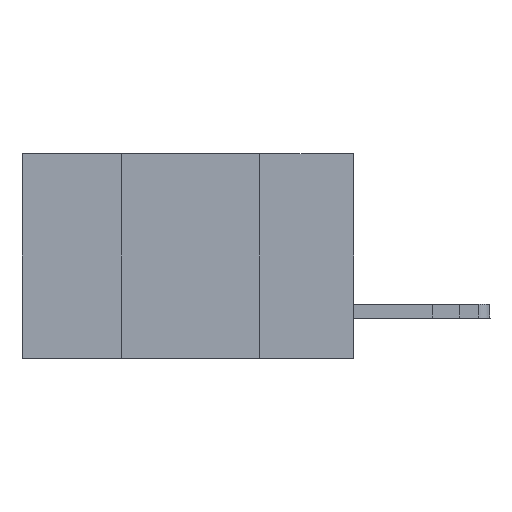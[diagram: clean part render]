
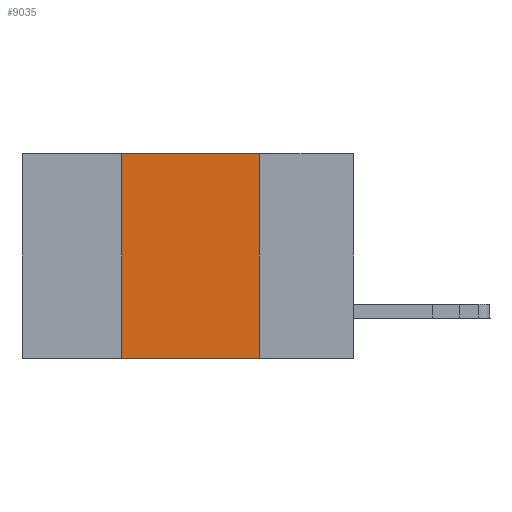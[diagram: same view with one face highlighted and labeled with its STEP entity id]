
A CAD part, left-side view. The second image highlights one B-rep face of the part: STEP entity #9035.
In plain terms, the highlighted planar face has unit normal (-1, 0, 0).
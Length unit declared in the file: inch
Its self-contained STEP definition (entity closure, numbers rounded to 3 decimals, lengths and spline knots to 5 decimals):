
#265 = DIRECTION ( 'NONE',  ( 0., -1., 0. ) ) ;
#642 = DIRECTION ( 'NONE',  ( 0., 0., -1. ) ) ;
#1886 = FACE_OUTER_BOUND ( 'NONE', #19502, .T. ) ;
#2486 = VECTOR ( 'NONE', #642, 39.37008 ) ;
#2557 = ORIENTED_EDGE ( 'NONE', *, *, #4417, .F. ) ;
#3030 = DIRECTION ( 'NONE',  ( 0., 0., 1. ) ) ;
#3118 = ORIENTED_EDGE ( 'NONE', *, *, #20024, .T. ) ;
#4417 = EDGE_CURVE ( 'NONE', #8883, #17363, #13126, .T. ) ;
#4745 = CARTESIAN_POINT ( 'NONE',  ( 0., 0.42, -0.37 ) ) ;
#5856 = EDGE_CURVE ( 'NONE', #7200, #8883, #7068, .T. ) ;
#5952 = LINE ( 'NONE', #14073, #2486 ) ;
#6340 = CARTESIAN_POINT ( 'NONE',  ( 0., 0.42, 0. ) ) ;
#6546 = VECTOR ( 'NONE', #3030, 39.37008 ) ;
#6786 = CARTESIAN_POINT ( 'NONE',  ( 0., 0.17, 0. ) ) ;
#7068 = LINE ( 'NONE', #6340, #6546 ) ;
#7200 = VERTEX_POINT ( 'NONE', #4745 ) ;
#7347 = CARTESIAN_POINT ( 'NONE',  ( 0., 0.17, -0.37 ) ) ;
#7489 = DIRECTION ( 'NONE',  ( 0., -1., 0. ) ) ;
#8713 = VECTOR ( 'NONE', #7489, 39.37008 ) ;
#8883 = VERTEX_POINT ( 'NONE', #19003 ) ;
#9035 = ADVANCED_FACE ( 'NONE', ( #1886 ), #17900, .F. ) ;
#9049 = AXIS2_PLACEMENT_3D ( 'NONE', #9645, #21223, #11288 ) ;
#9433 = VERTEX_POINT ( 'NONE', #7347 ) ;
#9645 = CARTESIAN_POINT ( 'NONE',  ( 0., 0.6, 0. ) ) ;
#9647 = VECTOR ( 'NONE', #265, 39.37008 ) ;
#10162 = LINE ( 'NONE', #12111, #9647 ) ;
#11288 = DIRECTION ( 'NONE',  ( 0., 0., -1. ) ) ;
#12111 = CARTESIAN_POINT ( 'NONE',  ( 0., 0.6, -0.37 ) ) ;
#12430 = CARTESIAN_POINT ( 'NONE',  ( 0., 0.6, 0. ) ) ;
#13126 = LINE ( 'NONE', #12430, #8713 ) ;
#13560 = EDGE_CURVE ( 'NONE', #17363, #9433, #5952, .T. ) ;
#14073 = CARTESIAN_POINT ( 'NONE',  ( 0., 0.17, 0. ) ) ;
#15883 = ORIENTED_EDGE ( 'NONE', *, *, #5856, .F. ) ;
#17363 = VERTEX_POINT ( 'NONE', #6786 ) ;
#17900 = PLANE ( 'NONE',  #9049 ) ;
#19003 = CARTESIAN_POINT ( 'NONE',  ( 0., 0.42, 0. ) ) ;
#19277 = ORIENTED_EDGE ( 'NONE', *, *, #13560, .F. ) ;
#19502 = EDGE_LOOP ( 'NONE', ( #19277, #2557, #15883, #3118 ) ) ;
#20024 = EDGE_CURVE ( 'NONE', #7200, #9433, #10162, .T. ) ;
#21223 = DIRECTION ( 'NONE',  ( 1., 0., 0. ) ) ;
